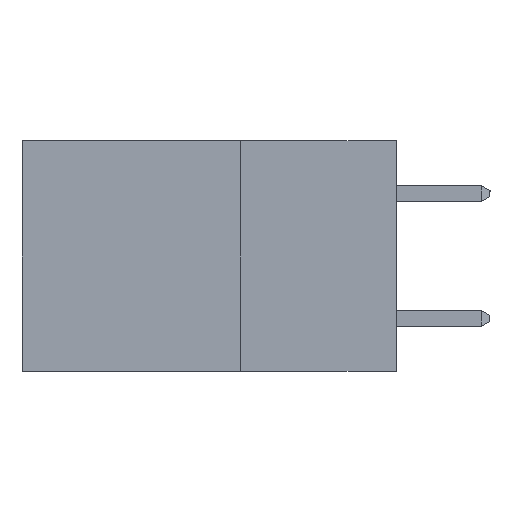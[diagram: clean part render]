
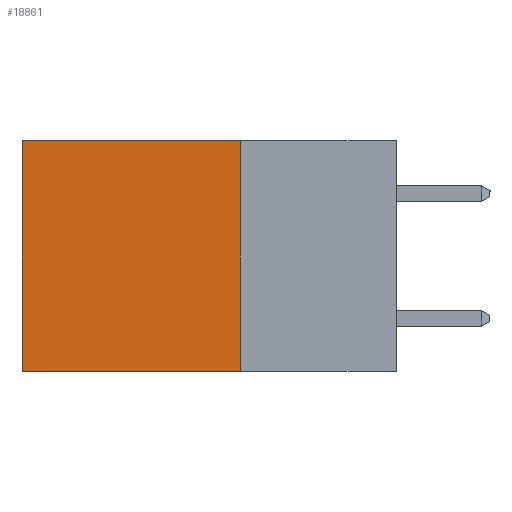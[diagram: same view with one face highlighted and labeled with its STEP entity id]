
A CAD part, left-side view. The second image highlights one B-rep face of the part: STEP entity #18861.
In plain terms, the highlighted planar face has unit normal (-1, 0, 0).
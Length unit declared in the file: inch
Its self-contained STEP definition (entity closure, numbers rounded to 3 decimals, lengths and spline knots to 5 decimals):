
#1707 = ORIENTED_EDGE ( 'NONE', *, *, #20884, .T. ) ;
#2959 = LINE ( 'NONE', #18778, #24270 ) ;
#3794 = EDGE_CURVE ( 'NONE', #19361, #8743, #2959, .T. ) ;
#3987 = ORIENTED_EDGE ( 'NONE', *, *, #5915, .T. ) ;
#4995 = CARTESIAN_POINT ( 'NONE',  ( 0.2615, 0.6, -0.37 ) ) ;
#5275 = FACE_OUTER_BOUND ( 'NONE', #13252, .T. ) ;
#5490 = ORIENTED_EDGE ( 'NONE', *, *, #3794, .F. ) ;
#5915 = EDGE_CURVE ( 'NONE', #19361, #15280, #24978, .T. ) ;
#6936 = DIRECTION ( 'NONE',  ( 0., 1., 0. ) ) ;
#8669 = LINE ( 'NONE', #18799, #24497 ) ;
#8743 = VERTEX_POINT ( 'NONE', #20053 ) ;
#12722 = EDGE_CURVE ( 'NONE', #8743, #13040, #25767, .T. ) ;
#12973 = DIRECTION ( 'NONE',  ( 0., 0., -1. ) ) ;
#13040 = VERTEX_POINT ( 'NONE', #4995 ) ;
#13252 = EDGE_LOOP ( 'NONE', ( #1707, #23952, #5490, #3987 ) ) ;
#13300 = DIRECTION ( 'NONE',  ( 0., 0., -1. ) ) ;
#13519 = CARTESIAN_POINT ( 'NONE',  ( 0.2615, 0.25, 0. ) ) ;
#15017 = CARTESIAN_POINT ( 'NONE',  ( 0.2615, 0.25, -0.37 ) ) ;
#15275 = PLANE ( 'NONE',  #24498 ) ;
#15280 = VERTEX_POINT ( 'NONE', #20735 ) ;
#18251 = DIRECTION ( 'NONE',  ( 0., 1., 0. ) ) ;
#18411 = DIRECTION ( 'NONE',  ( 0., 0., -1. ) ) ;
#18778 = CARTESIAN_POINT ( 'NONE',  ( 0.2615, 0.25, -0.37 ) ) ;
#18799 = CARTESIAN_POINT ( 'NONE',  ( 0.2615, 0.6, -0.37 ) ) ;
#18861 = ADVANCED_FACE ( 'NONE', ( #5275 ), #15275, .F. ) ;
#19019 = VECTOR ( 'NONE', #6936, 39.37008 ) ;
#19361 = VERTEX_POINT ( 'NONE', #13519 ) ;
#20053 = CARTESIAN_POINT ( 'NONE',  ( 0.2615, 0.25, -0.37 ) ) ;
#20735 = CARTESIAN_POINT ( 'NONE',  ( 0.2615, 0.6, 0. ) ) ;
#20884 = EDGE_CURVE ( 'NONE', #15280, #13040, #8669, .T. ) ;
#21924 = CARTESIAN_POINT ( 'NONE',  ( 0.2615, 0.25, -0.37 ) ) ;
#22736 = CARTESIAN_POINT ( 'NONE',  ( 0.2615, 0.25, 0. ) ) ;
#23074 = DIRECTION ( 'NONE',  ( 1., 0., 0. ) ) ;
#23952 = ORIENTED_EDGE ( 'NONE', *, *, #12722, .F. ) ;
#24230 = VECTOR ( 'NONE', #18251, 39.37008 ) ;
#24270 = VECTOR ( 'NONE', #12973, 39.37008 ) ;
#24497 = VECTOR ( 'NONE', #18411, 39.37008 ) ;
#24498 = AXIS2_PLACEMENT_3D ( 'NONE', #15017, #23074, #13300 ) ;
#24978 = LINE ( 'NONE', #22736, #19019 ) ;
#25767 = LINE ( 'NONE', #21924, #24230 ) ;
